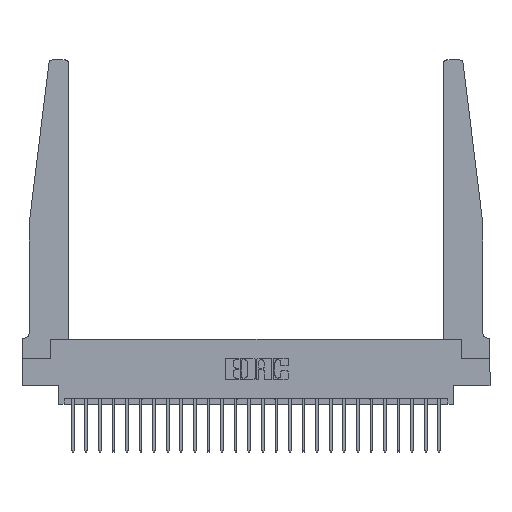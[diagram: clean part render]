
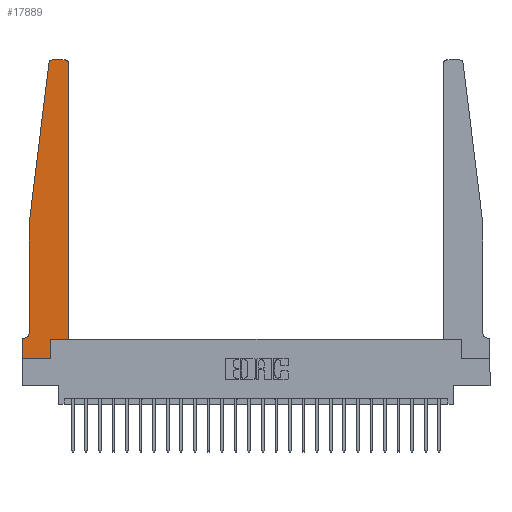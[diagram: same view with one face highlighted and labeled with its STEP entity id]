
A CAD part, top view. The second image highlights one B-rep face of the part: STEP entity #17889.
In plain terms, the highlighted planar face has unit normal (0, 0, 1).
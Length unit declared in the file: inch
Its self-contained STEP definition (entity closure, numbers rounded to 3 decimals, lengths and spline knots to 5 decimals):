
#42 = CARTESIAN_POINT ( 'NONE',  ( 0.2605, 0., 0.37 ) ) ;
#154 = VERTEX_POINT ( 'NONE', #24369 ) ;
#836 = EDGE_CURVE ( 'NONE', #21500, #23601, #19090, .T. ) ;
#929 = CIRCLE ( 'NONE', #19066, 0.05 ) ;
#968 = FACE_OUTER_BOUND ( 'NONE', #8799, .T. ) ;
#1185 = LINE ( 'NONE', #11772, #15601 ) ;
#1642 = VECTOR ( 'NONE', #12105, 39.37008 ) ;
#2215 = VECTOR ( 'NONE', #16871, 39.37008 ) ;
#2282 = LINE ( 'NONE', #6236, #1642 ) ;
#2778 = VECTOR ( 'NONE', #18554, 39.37008 ) ;
#2932 = ORIENTED_EDGE ( 'NONE', *, *, #22541, .T. ) ;
#2987 = CARTESIAN_POINT ( 'NONE',  ( 0.425, 0.18, 0.37 ) ) ;
#3089 = DIRECTION ( 'NONE',  ( 0., -1., 0. ) ) ;
#3168 = AXIS2_PLACEMENT_3D ( 'NONE', #20131, #8545, #22019 ) ;
#4147 = VERTEX_POINT ( 'NONE', #20922 ) ;
#4509 = EDGE_CURVE ( 'NONE', #13334, #21500, #13018, .T. ) ;
#5051 = LINE ( 'NONE', #14236, #19942 ) ;
#5879 = VERTEX_POINT ( 'NONE', #14813 ) ;
#5943 = CARTESIAN_POINT ( 'NONE',  ( 0.065, 1.25, 0.37 ) ) ;
#6034 = DIRECTION ( 'NONE',  ( 0., 0., -1. ) ) ;
#6236 = CARTESIAN_POINT ( 'NONE',  ( 0.2605, 0.18, 0.37 ) ) ;
#6257 = ORIENTED_EDGE ( 'NONE', *, *, #14401, .T. ) ;
#6297 = EDGE_CURVE ( 'NONE', #24271, #10379, #21916, .T. ) ;
#6311 = VECTOR ( 'NONE', #3089, 39.37008 ) ;
#6528 = EDGE_CURVE ( 'NONE', #10379, #8983, #22805, .T. ) ;
#6637 = VECTOR ( 'NONE', #15895, 39.37008 ) ;
#7312 = VERTEX_POINT ( 'NONE', #42 ) ;
#7449 = DIRECTION ( 'NONE',  ( 1., 0., 0. ) ) ;
#7795 = CARTESIAN_POINT ( 'NONE',  ( 0.425, 2.72, 0.37 ) ) ;
#7827 = ORIENTED_EDGE ( 'NONE', *, *, #12895, .T. ) ;
#7970 = EDGE_CURVE ( 'NONE', #7312, #4147, #2282, .T. ) ;
#7996 = LINE ( 'NONE', #2987, #2778 ) ;
#8245 = DIRECTION ( 'NONE',  ( -1., 0., 0. ) ) ;
#8306 = CARTESIAN_POINT ( 'NONE',  ( 0.395, 2.72, 0.37 ) ) ;
#8401 = VECTOR ( 'NONE', #8245, 39.37008 ) ;
#8545 = DIRECTION ( 'NONE',  ( 0., 0., 1. ) ) ;
#8755 = VECTOR ( 'NONE', #11237, 39.37008 ) ;
#8799 = EDGE_LOOP ( 'NONE', ( #21994, #7827, #16947, #2932, #24056, #22285, #22891, #6257, #12129, #12204, #22358, #13417 ) ) ;
#8935 = EDGE_CURVE ( 'NONE', #9745, #13334, #929, .T. ) ;
#8983 = VERTEX_POINT ( 'NONE', #17791 ) ;
#9745 = VERTEX_POINT ( 'NONE', #21734 ) ;
#10298 = AXIS2_PLACEMENT_3D ( 'NONE', #24677, #19111, #7449 ) ;
#10305 = DIRECTION ( 'NONE',  ( 1., 0., 0. ) ) ;
#10379 = VERTEX_POINT ( 'NONE', #14289 ) ;
#10888 = CARTESIAN_POINT ( 'NONE',  ( 0.065, 1.25, 0.37 ) ) ;
#11100 = EDGE_CURVE ( 'NONE', #154, #24271, #7996, .T. ) ;
#11237 = DIRECTION ( 'NONE',  ( 0., -1., 0. ) ) ;
#11772 = CARTESIAN_POINT ( 'NONE',  ( 0.425, 0.18, 0.37 ) ) ;
#12046 = CARTESIAN_POINT ( 'NONE',  ( 0.065, 1.25, 0.37 ) ) ;
#12105 = DIRECTION ( 'NONE',  ( 0., 1., 0. ) ) ;
#12129 = ORIENTED_EDGE ( 'NONE', *, *, #7970, .T. ) ;
#12204 = ORIENTED_EDGE ( 'NONE', *, *, #20120, .T. ) ;
#12213 = CIRCLE ( 'NONE', #3168, 0.03 ) ;
#12895 = EDGE_CURVE ( 'NONE', #8983, #5879, #12213, .T. ) ;
#12986 = CARTESIAN_POINT ( 'NONE',  ( 0., 0., 0.37 ) ) ;
#13018 = LINE ( 'NONE', #21803, #8401 ) ;
#13334 = VERTEX_POINT ( 'NONE', #17623 ) ;
#13417 = ORIENTED_EDGE ( 'NONE', *, *, #6297, .T. ) ;
#14236 = CARTESIAN_POINT ( 'NONE',  ( 0., 0., 0.37 ) ) ;
#14289 = CARTESIAN_POINT ( 'NONE',  ( 0.395, 2.75, 0.37 ) ) ;
#14401 = EDGE_CURVE ( 'NONE', #23601, #7312, #5051, .T. ) ;
#14813 = CARTESIAN_POINT ( 'NONE',  ( 0.24675, 2.72367, 0.37 ) ) ;
#15601 = VECTOR ( 'NONE', #17573, 39.37008 ) ;
#15743 = CARTESIAN_POINT ( 'NONE',  ( 0., 0.1875, 0.37 ) ) ;
#15895 = DIRECTION ( 'NONE',  ( -0.122, -0.992, 0. ) ) ;
#16871 = DIRECTION ( 'NONE',  ( -1., 0., 0. ) ) ;
#16947 = ORIENTED_EDGE ( 'NONE', *, *, #21576, .T. ) ;
#17159 = PLANE ( 'NONE',  #10298 ) ;
#17573 = DIRECTION ( 'NONE',  ( 1., 0., 0. ) ) ;
#17623 = CARTESIAN_POINT ( 'NONE',  ( 0.015, 0.1875, 0.37 ) ) ;
#17713 = CARTESIAN_POINT ( 'NONE',  ( 0.015, 0.2375, 0.37 ) ) ;
#17791 = CARTESIAN_POINT ( 'NONE',  ( 0.27653, 2.75, 0.37 ) ) ;
#17889 = ADVANCED_FACE ( 'NONE', ( #968 ), #17159, .T. ) ;
#18104 = DIRECTION ( 'NONE',  ( 1., 0., 0. ) ) ;
#18554 = DIRECTION ( 'NONE',  ( 0., 1., 0. ) ) ;
#19066 = AXIS2_PLACEMENT_3D ( 'NONE', #17713, #6034, #19655 ) ;
#19090 = LINE ( 'NONE', #24578, #8755 ) ;
#19111 = DIRECTION ( 'NONE',  ( 0., 0., 1. ) ) ;
#19655 = DIRECTION ( 'NONE',  ( -1., 0., 0. ) ) ;
#19942 = VECTOR ( 'NONE', #18104, 39.37008 ) ;
#20120 = EDGE_CURVE ( 'NONE', #4147, #154, #1185, .T. ) ;
#20131 = CARTESIAN_POINT ( 'NONE',  ( 0.27653, 2.72, 0.37 ) ) ;
#20639 = CARTESIAN_POINT ( 'NONE',  ( 0.25, 2.75, 0.37 ) ) ;
#20922 = CARTESIAN_POINT ( 'NONE',  ( 0.2605, 0.18, 0.37 ) ) ;
#21500 = VERTEX_POINT ( 'NONE', #15743 ) ;
#21576 = EDGE_CURVE ( 'NONE', #5879, #23180, #22642, .T. ) ;
#21734 = CARTESIAN_POINT ( 'NONE',  ( 0.065, 0.2375, 0.37 ) ) ;
#21745 = LINE ( 'NONE', #10888, #6311 ) ;
#21787 = DIRECTION ( 'NONE',  ( 0., 0., 1. ) ) ;
#21803 = CARTESIAN_POINT ( 'NONE',  ( 0.065, 0.1875, 0.37 ) ) ;
#21916 = CIRCLE ( 'NONE', #23588, 0.03 ) ;
#21994 = ORIENTED_EDGE ( 'NONE', *, *, #6528, .T. ) ;
#22019 = DIRECTION ( 'NONE',  ( 1., 0., 0. ) ) ;
#22285 = ORIENTED_EDGE ( 'NONE', *, *, #4509, .T. ) ;
#22358 = ORIENTED_EDGE ( 'NONE', *, *, #11100, .T. ) ;
#22541 = EDGE_CURVE ( 'NONE', #23180, #9745, #21745, .T. ) ;
#22642 = LINE ( 'NONE', #12046, #6637 ) ;
#22805 = LINE ( 'NONE', #20639, #2215 ) ;
#22891 = ORIENTED_EDGE ( 'NONE', *, *, #836, .T. ) ;
#23180 = VERTEX_POINT ( 'NONE', #5943 ) ;
#23588 = AXIS2_PLACEMENT_3D ( 'NONE', #8306, #21787, #10305 ) ;
#23601 = VERTEX_POINT ( 'NONE', #12986 ) ;
#24056 = ORIENTED_EDGE ( 'NONE', *, *, #8935, .T. ) ;
#24271 = VERTEX_POINT ( 'NONE', #7795 ) ;
#24369 = CARTESIAN_POINT ( 'NONE',  ( 0.425, 0.18, 0.37 ) ) ;
#24578 = CARTESIAN_POINT ( 'NONE',  ( 0., 0., 0.37 ) ) ;
#24677 = CARTESIAN_POINT ( 'NONE',  ( 0., 0.1875, 0.37 ) ) ;
